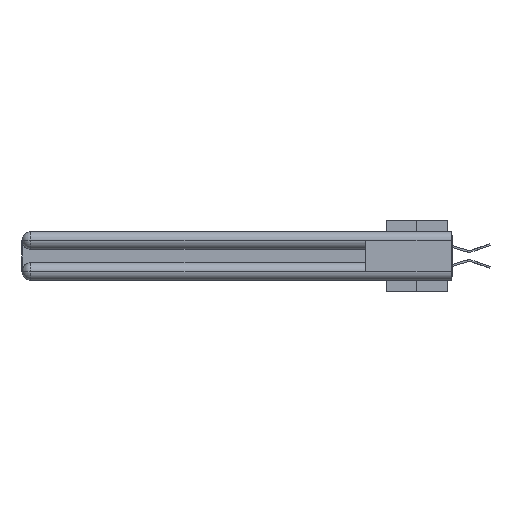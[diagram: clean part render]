
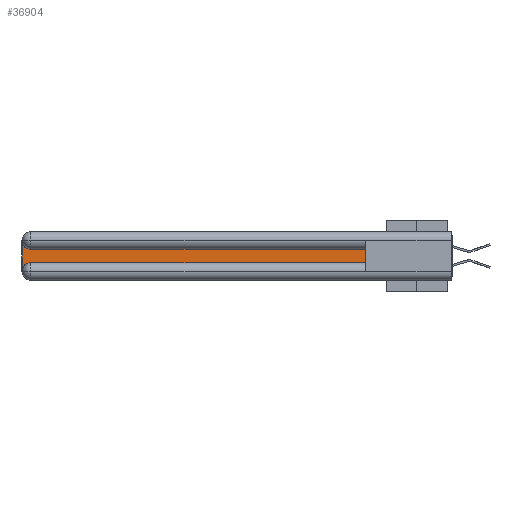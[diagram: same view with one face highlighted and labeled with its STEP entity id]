
A CAD part, left-side view. The second image highlights one B-rep face of the part: STEP entity #36904.
In plain terms, the highlighted planar face has unit normal (-1, 0, 0).
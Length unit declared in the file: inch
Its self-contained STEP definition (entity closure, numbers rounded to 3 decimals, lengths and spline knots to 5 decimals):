
#75 = EDGE_CURVE ( 'NONE', #16796, #13425, #18690, .T. ) ;
#3358 = EDGE_CURVE ( 'NONE', #27356, #35671, #20552, .T. ) ;
#4200 = DIRECTION ( 'NONE',  ( 0., 1., 0. ) ) ;
#4827 = AXIS2_PLACEMENT_3D ( 'NONE', #27477, #9849, #20516 ) ;
#5688 = EDGE_LOOP ( 'NONE', ( #12442, #11126, #37883, #7401, #37823, #40903 ) ) ;
#6998 = DIRECTION ( 'NONE',  ( 1., 0., 0. ) ) ;
#7144 = DIRECTION ( 'NONE',  ( 0., 0., -1. ) ) ;
#7401 = ORIENTED_EDGE ( 'NONE', *, *, #38074, .T. ) ;
#7751 = CARTESIAN_POINT ( 'NONE',  ( 0.075, 2.94, -0.2175 ) ) ;
#9561 = VECTOR ( 'NONE', #32225, 39.37008 ) ;
#9849 = DIRECTION ( 'NONE',  ( 1., 0., 0. ) ) ;
#10201 = EDGE_CURVE ( 'NONE', #13425, #27356, #29115, .T. ) ;
#10460 = CARTESIAN_POINT ( 'NONE',  ( 0.075, 2.94, -0.1225 ) ) ;
#11126 = ORIENTED_EDGE ( 'NONE', *, *, #10201, .T. ) ;
#11337 = AXIS2_PLACEMENT_3D ( 'NONE', #17156, #6998, #7144 ) ;
#12442 = ORIENTED_EDGE ( 'NONE', *, *, #75, .T. ) ;
#13167 = DIRECTION ( 'NONE',  ( 0., 0., -1. ) ) ;
#13425 = VERTEX_POINT ( 'NONE', #10460 ) ;
#13669 = PLANE ( 'NONE',  #4827 ) ;
#15218 = VERTEX_POINT ( 'NONE', #29467 ) ;
#16796 = VERTEX_POINT ( 'NONE', #26674 ) ;
#17156 = CARTESIAN_POINT ( 'NONE',  ( 0.075, 2.94, -0.0625 ) ) ;
#18644 = DIRECTION ( 'NONE',  ( 1., 0., 0. ) ) ;
#18690 = LINE ( 'NONE', #24659, #22944 ) ;
#20516 = DIRECTION ( 'NONE',  ( 0., 0., -1. ) ) ;
#20552 = LINE ( 'NONE', #37918, #30051 ) ;
#22944 = VECTOR ( 'NONE', #4200, 39.37008 ) ;
#24262 = CARTESIAN_POINT ( 'NONE',  ( 0.075, 2.94, -0.2775 ) ) ;
#24659 = CARTESIAN_POINT ( 'NONE',  ( 0.075, 0.6, -0.1225 ) ) ;
#26532 = LINE ( 'NONE', #43328, #35513 ) ;
#26674 = CARTESIAN_POINT ( 'NONE',  ( 0.075, 0.6, -0.1225 ) ) ;
#26986 = EDGE_CURVE ( 'NONE', #41696, #15218, #26532, .T. ) ;
#27356 = VERTEX_POINT ( 'NONE', #27671 ) ;
#27394 = EDGE_CURVE ( 'NONE', #15218, #16796, #28629, .T. ) ;
#27477 = CARTESIAN_POINT ( 'NONE',  ( 0.075, 3., -0.1225 ) ) ;
#27671 = CARTESIAN_POINT ( 'NONE',  ( 0.075, 3., -0.0625 ) ) ;
#28268 = CARTESIAN_POINT ( 'NONE',  ( 0.075, 0.6, -0.2175 ) ) ;
#28629 = LINE ( 'NONE', #28268, #9561 ) ;
#29115 = CIRCLE ( 'NONE', #11337, 0.06 ) ;
#29467 = CARTESIAN_POINT ( 'NONE',  ( 0.075, 0.6, -0.2175 ) ) ;
#30051 = VECTOR ( 'NONE', #38515, 39.37008 ) ;
#32225 = DIRECTION ( 'NONE',  ( 0., 0., 1. ) ) ;
#33390 = CARTESIAN_POINT ( 'NONE',  ( 0.075, 3., -0.2775 ) ) ;
#33406 = DIRECTION ( 'NONE',  ( 0., -1., 0. ) ) ;
#34621 = AXIS2_PLACEMENT_3D ( 'NONE', #24262, #18644, #13167 ) ;
#34724 = FACE_OUTER_BOUND ( 'NONE', #5688, .T. ) ;
#35513 = VECTOR ( 'NONE', #33406, 39.37008 ) ;
#35671 = VERTEX_POINT ( 'NONE', #33390 ) ;
#36904 = ADVANCED_FACE ( 'NONE', ( #34724 ), #13669, .F. ) ;
#37823 = ORIENTED_EDGE ( 'NONE', *, *, #26986, .T. ) ;
#37883 = ORIENTED_EDGE ( 'NONE', *, *, #3358, .T. ) ;
#37918 = CARTESIAN_POINT ( 'NONE',  ( 0.075, 3., -0.2175 ) ) ;
#38074 = EDGE_CURVE ( 'NONE', #35671, #41696, #43166, .T. ) ;
#38515 = DIRECTION ( 'NONE',  ( 0., 0., -1. ) ) ;
#40903 = ORIENTED_EDGE ( 'NONE', *, *, #27394, .T. ) ;
#41696 = VERTEX_POINT ( 'NONE', #7751 ) ;
#43166 = CIRCLE ( 'NONE', #34621, 0.06 ) ;
#43328 = CARTESIAN_POINT ( 'NONE',  ( 0.075, 0.6, -0.2175 ) ) ;
